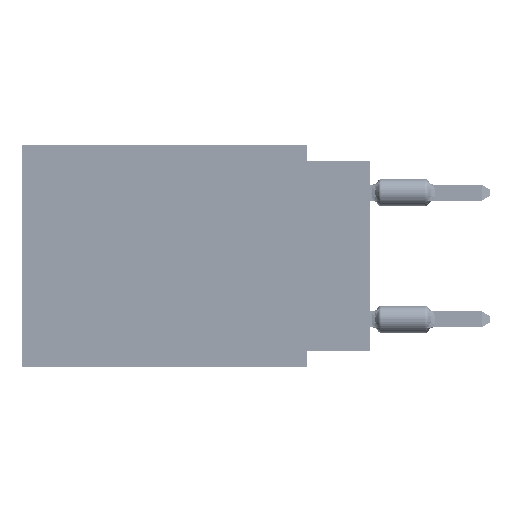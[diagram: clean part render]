
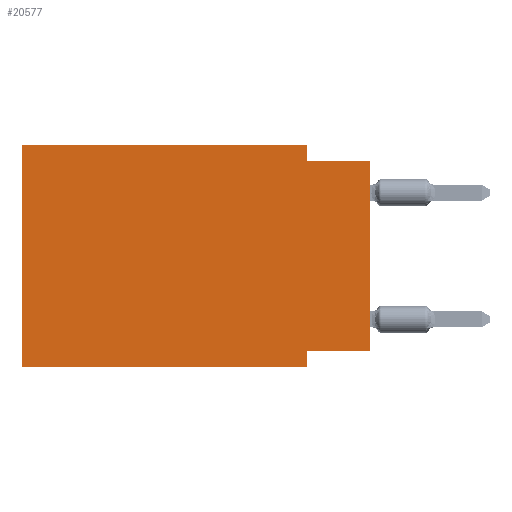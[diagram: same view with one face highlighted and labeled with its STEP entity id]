
A CAD part, left-side view. The second image highlights one B-rep face of the part: STEP entity #20577.
In plain terms, the highlighted planar face has unit normal (-1, 0, 0).
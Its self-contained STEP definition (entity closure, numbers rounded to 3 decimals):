
#247 = EDGE_CURVE ( 'NONE', #20483, #61058, #16545, .T. ) ;
#645 = ORIENTED_EDGE ( 'NONE', *, *, #53125, .T. ) ;
#1383 = CARTESIAN_POINT ( 'NONE',  ( 0., 0., -0.635 ) ) ;
#3998 = ORIENTED_EDGE ( 'NONE', *, *, #59021, .F. ) ;
#4833 = CARTESIAN_POINT ( 'NONE',  ( 0., 2.54, -8.89 ) ) ;
#5022 = VERTEX_POINT ( 'NONE', #54522 ) ;
#7401 = DIRECTION ( 'NONE',  ( 0., -1., 0. ) ) ;
#7735 = CARTESIAN_POINT ( 'NONE',  ( 0., 0., -8.255 ) ) ;
#11752 = VECTOR ( 'NONE', #41971, 1000. ) ;
#12390 = VECTOR ( 'NONE', #60771, 1000. ) ;
#13067 = PLANE ( 'NONE',  #34330 ) ;
#13249 = ORIENTED_EDGE ( 'NONE', *, *, #45313, .F. ) ;
#14495 = DIRECTION ( 'NONE',  ( 0., -1., 0. ) ) ;
#15447 = VERTEX_POINT ( 'NONE', #32016 ) ;
#15574 = LINE ( 'NONE', #4833, #57397 ) ;
#16429 = EDGE_CURVE ( 'NONE', #59128, #58484, #32807, .T. ) ;
#16545 = LINE ( 'NONE', #36440, #63976 ) ;
#17816 = CARTESIAN_POINT ( 'NONE',  ( 0., 13.97, 0. ) ) ;
#18432 = CARTESIAN_POINT ( 'NONE',  ( 0., 13.97, -8.89 ) ) ;
#19691 = EDGE_CURVE ( 'NONE', #59059, #15447, #53948, .T. ) ;
#19899 = EDGE_CURVE ( 'NONE', #47586, #5022, #54590, .T. ) ;
#20483 = VERTEX_POINT ( 'NONE', #62940 ) ;
#20577 = ADVANCED_FACE ( 'NONE', ( #28054 ), #13067, .F. ) ;
#20746 = DIRECTION ( 'NONE',  ( 0., 0., 1. ) ) ;
#22852 = DIRECTION ( 'NONE',  ( 0., 0., -1. ) ) ;
#27065 = ORIENTED_EDGE ( 'NONE', *, *, #16429, .F. ) ;
#27163 = EDGE_LOOP ( 'NONE', ( #645, #40562, #3998, #38900, #47291, #28112, #13249, #27065 ) ) ;
#28054 = FACE_OUTER_BOUND ( 'NONE', #27163, .T. ) ;
#28112 = ORIENTED_EDGE ( 'NONE', *, *, #19691, .T. ) ;
#30860 = VECTOR ( 'NONE', #36453, 1000. ) ;
#32016 = CARTESIAN_POINT ( 'NONE',  ( 0., 2.54, -8.89 ) ) ;
#32248 = VECTOR ( 'NONE', #20746, 1000. ) ;
#32807 = LINE ( 'NONE', #52995, #55698 ) ;
#33410 = CARTESIAN_POINT ( 'NONE',  ( 0., 2.54, -8.255 ) ) ;
#34330 = AXIS2_PLACEMENT_3D ( 'NONE', #47949, #52518, #22852 ) ;
#36440 = CARTESIAN_POINT ( 'NONE',  ( 0., 0., -0.635 ) ) ;
#36453 = DIRECTION ( 'NONE',  ( 0., 0., -1. ) ) ;
#37389 = VECTOR ( 'NONE', #14495, 1000. ) ;
#38900 = ORIENTED_EDGE ( 'NONE', *, *, #19899, .F. ) ;
#40354 = DIRECTION ( 'NONE',  ( 0., 0., -1. ) ) ;
#40562 = ORIENTED_EDGE ( 'NONE', *, *, #247, .F. ) ;
#40700 = LINE ( 'NONE', #49280, #30860 ) ;
#41971 = DIRECTION ( 'NONE',  ( 0., 0., 1. ) ) ;
#44489 = CARTESIAN_POINT ( 'NONE',  ( 0., 13.97, 0. ) ) ;
#45313 = EDGE_CURVE ( 'NONE', #58484, #15447, #15574, .T. ) ;
#47291 = ORIENTED_EDGE ( 'NONE', *, *, #56743, .F. ) ;
#47586 = VERTEX_POINT ( 'NONE', #52890 ) ;
#47949 = CARTESIAN_POINT ( 'NONE',  ( 0., 13.97, 0. ) ) ;
#49280 = CARTESIAN_POINT ( 'NONE',  ( 0., 2.54, 0. ) ) ;
#49473 = LINE ( 'NONE', #54353, #32248 ) ;
#51737 = LINE ( 'NONE', #17816, #11752 ) ;
#52518 = DIRECTION ( 'NONE',  ( 1., 0., 0. ) ) ;
#52890 = CARTESIAN_POINT ( 'NONE',  ( 0., 13.97, 0. ) ) ;
#52995 = CARTESIAN_POINT ( 'NONE',  ( 0., 0., -8.255 ) ) ;
#53125 = EDGE_CURVE ( 'NONE', #59128, #61058, #49473, .T. ) ;
#53948 = LINE ( 'NONE', #18432, #37389 ) ;
#54353 = CARTESIAN_POINT ( 'NONE',  ( 0., 0., 0. ) ) ;
#54522 = CARTESIAN_POINT ( 'NONE',  ( 0., 2.54, 0. ) ) ;
#54590 = LINE ( 'NONE', #44489, #12390 ) ;
#55698 = VECTOR ( 'NONE', #63107, 1000. ) ;
#56743 = EDGE_CURVE ( 'NONE', #59059, #47586, #51737, .T. ) ;
#57397 = VECTOR ( 'NONE', #40354, 1000. ) ;
#58484 = VERTEX_POINT ( 'NONE', #33410 ) ;
#59021 = EDGE_CURVE ( 'NONE', #5022, #20483, #40700, .T. ) ;
#59059 = VERTEX_POINT ( 'NONE', #60909 ) ;
#59128 = VERTEX_POINT ( 'NONE', #7735 ) ;
#60771 = DIRECTION ( 'NONE',  ( 0., -1., 0. ) ) ;
#60909 = CARTESIAN_POINT ( 'NONE',  ( 0., 13.97, -8.89 ) ) ;
#61058 = VERTEX_POINT ( 'NONE', #1383 ) ;
#62940 = CARTESIAN_POINT ( 'NONE',  ( 0., 2.54, -0.635 ) ) ;
#63107 = DIRECTION ( 'NONE',  ( 0., 1., 0. ) ) ;
#63976 = VECTOR ( 'NONE', #7401, 1000. ) ;
